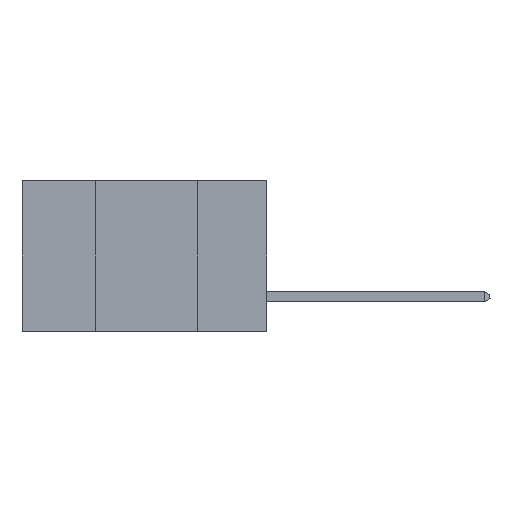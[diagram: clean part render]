
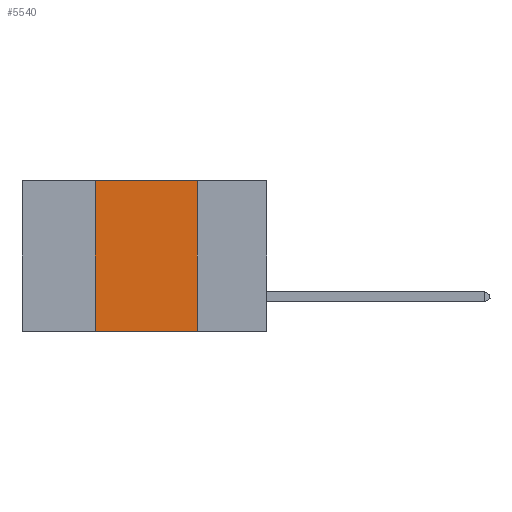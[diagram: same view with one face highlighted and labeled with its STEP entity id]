
A CAD part, left-side view. The second image highlights one B-rep face of the part: STEP entity #5540.
In plain terms, the highlighted planar face has unit normal (-1, 0, 0).
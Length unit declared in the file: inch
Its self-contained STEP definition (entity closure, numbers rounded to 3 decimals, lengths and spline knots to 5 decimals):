
#158 = EDGE_CURVE ( 'NONE', #221, #4461, #2574, .T. ) ;
#177 = LINE ( 'NONE', #11831, #6267 ) ;
#221 = VERTEX_POINT ( 'NONE', #6201 ) ;
#601 = EDGE_CURVE ( 'NONE', #8857, #221, #3936, .T. ) ;
#1258 = ORIENTED_EDGE ( 'NONE', *, *, #3965, .T. ) ;
#1571 = DIRECTION ( 'NONE',  ( 0., 0., -1. ) ) ;
#1782 = CARTESIAN_POINT ( 'NONE',  ( 0., 0.6, 0. ) ) ;
#1933 = CARTESIAN_POINT ( 'NONE',  ( 0., 0.42, 0. ) ) ;
#2175 = VERTEX_POINT ( 'NONE', #6760 ) ;
#2574 = LINE ( 'NONE', #10862, #12331 ) ;
#2755 = CARTESIAN_POINT ( 'NONE',  ( 0., 0.6, -0.37 ) ) ;
#2789 = VECTOR ( 'NONE', #9583, 39.37008 ) ;
#3043 = AXIS2_PLACEMENT_3D ( 'NONE', #12244, #11371, #1571 ) ;
#3936 = LINE ( 'NONE', #1782, #5291 ) ;
#3965 = EDGE_CURVE ( 'NONE', #2175, #4461, #4603, .T. ) ;
#4146 = ORIENTED_EDGE ( 'NONE', *, *, #601, .F. ) ;
#4461 = VERTEX_POINT ( 'NONE', #9461 ) ;
#4603 = LINE ( 'NONE', #2755, #2789 ) ;
#5291 = VECTOR ( 'NONE', #8456, 39.37008 ) ;
#5540 = ADVANCED_FACE ( 'NONE', ( #8739 ), #8483, .F. ) ;
#6201 = CARTESIAN_POINT ( 'NONE',  ( 0., 0.17, 0. ) ) ;
#6267 = VECTOR ( 'NONE', #9893, 39.37008 ) ;
#6760 = CARTESIAN_POINT ( 'NONE',  ( 0., 0.42, -0.37 ) ) ;
#7231 = EDGE_CURVE ( 'NONE', #2175, #8857, #177, .T. ) ;
#8131 = DIRECTION ( 'NONE',  ( 0., 0., -1. ) ) ;
#8456 = DIRECTION ( 'NONE',  ( 0., -1., 0. ) ) ;
#8483 = PLANE ( 'NONE',  #3043 ) ;
#8666 = ORIENTED_EDGE ( 'NONE', *, *, #158, .F. ) ;
#8739 = FACE_OUTER_BOUND ( 'NONE', #12452, .T. ) ;
#8857 = VERTEX_POINT ( 'NONE', #1933 ) ;
#9461 = CARTESIAN_POINT ( 'NONE',  ( 0., 0.17, -0.37 ) ) ;
#9583 = DIRECTION ( 'NONE',  ( 0., -1., 0. ) ) ;
#9893 = DIRECTION ( 'NONE',  ( 0., 0., 1. ) ) ;
#10862 = CARTESIAN_POINT ( 'NONE',  ( 0., 0.17, 0. ) ) ;
#10961 = ORIENTED_EDGE ( 'NONE', *, *, #7231, .F. ) ;
#11371 = DIRECTION ( 'NONE',  ( 1., 0., 0. ) ) ;
#11831 = CARTESIAN_POINT ( 'NONE',  ( 0., 0.42, 0. ) ) ;
#12244 = CARTESIAN_POINT ( 'NONE',  ( 0., 0.6, 0. ) ) ;
#12331 = VECTOR ( 'NONE', #8131, 39.37008 ) ;
#12452 = EDGE_LOOP ( 'NONE', ( #8666, #4146, #10961, #1258 ) ) ;
